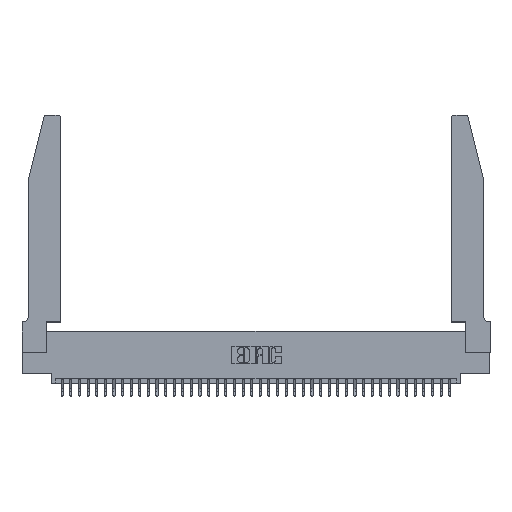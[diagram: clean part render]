
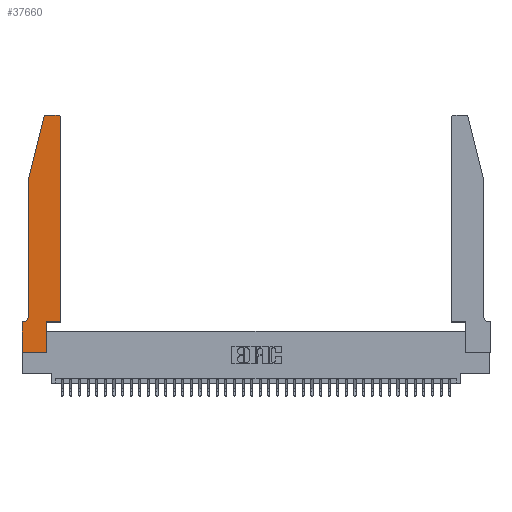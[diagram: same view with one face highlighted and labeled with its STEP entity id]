
A CAD part, top view. The second image highlights one B-rep face of the part: STEP entity #37660.
In plain terms, the highlighted planar face has unit normal (0, 0, 1).
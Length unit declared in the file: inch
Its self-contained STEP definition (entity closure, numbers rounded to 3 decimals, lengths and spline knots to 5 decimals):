
#400 = EDGE_CURVE ( 'NONE', #38491, #24697, #34433, .T. ) ;
#1029 = ORIENTED_EDGE ( 'NONE', *, *, #28770, .T. ) ;
#1080 = LINE ( 'NONE', #39253, #33537 ) ;
#1335 = ORIENTED_EDGE ( 'NONE', *, *, #400, .T. ) ;
#1460 = EDGE_CURVE ( 'NONE', #26523, #8110, #8749, .T. ) ;
#1793 = CIRCLE ( 'NONE', #32976, 0.03 ) ;
#2580 = DIRECTION ( 'NONE',  ( -1., 0., 0. ) ) ;
#3582 = ORIENTED_EDGE ( 'NONE', *, *, #23588, .T. ) ;
#4077 = CARTESIAN_POINT ( 'NONE',  ( 0.284, 2.75, 0.37 ) ) ;
#4135 = LINE ( 'NONE', #27536, #13419 ) ;
#4335 = VERTEX_POINT ( 'NONE', #8247 ) ;
#4940 = CARTESIAN_POINT ( 'NONE',  ( 0., 0., 0.37 ) ) ;
#5087 = ORIENTED_EDGE ( 'NONE', *, *, #16750, .T. ) ;
#5762 = DIRECTION ( 'NONE',  ( 0., 1., 0. ) ) ;
#6700 = CARTESIAN_POINT ( 'NONE',  ( 0.25487, 2.72718, 0.37 ) ) ;
#7778 = EDGE_CURVE ( 'NONE', #38697, #26523, #26146, .T. ) ;
#8110 = VERTEX_POINT ( 'NONE', #27173 ) ;
#8247 = CARTESIAN_POINT ( 'NONE',  ( 0., 0.35, 0.37 ) ) ;
#8749 = LINE ( 'NONE', #33118, #11166 ) ;
#8798 = EDGE_CURVE ( 'NONE', #30592, #4335, #38366, .T. ) ;
#8995 = CARTESIAN_POINT ( 'NONE',  ( 0., 0., 0.37 ) ) ;
#9205 = VERTEX_POINT ( 'NONE', #36816 ) ;
#9849 = ORIENTED_EDGE ( 'NONE', *, *, #14653, .T. ) ;
#10394 = VECTOR ( 'NONE', #10455, 39.37008 ) ;
#10455 = DIRECTION ( 'NONE',  ( 0., -1., 0. ) ) ;
#10794 = DIRECTION ( 'NONE',  ( -1., 0., 0. ) ) ;
#11007 = EDGE_CURVE ( 'NONE', #28979, #38697, #1793, .T. ) ;
#11166 = VECTOR ( 'NONE', #23547, 39.37008 ) ;
#11453 = EDGE_CURVE ( 'NONE', #8110, #30592, #21383, .T. ) ;
#11555 = CARTESIAN_POINT ( 'NONE',  ( 0.2865, 0.35, 0.37 ) ) ;
#11758 = AXIS2_PLACEMENT_3D ( 'NONE', #34910, #22427, #25447 ) ;
#12057 = CARTESIAN_POINT ( 'NONE',  ( 0.2865, 0., 0.37 ) ) ;
#12674 = FACE_OUTER_BOUND ( 'NONE', #14682, .T. ) ;
#12895 = VECTOR ( 'NONE', #31483, 39.37008 ) ;
#13020 = VECTOR ( 'NONE', #16744, 39.37008 ) ;
#13419 = VECTOR ( 'NONE', #37011, 39.37008 ) ;
#14029 = CIRCLE ( 'NONE', #29671, 0.03 ) ;
#14653 = EDGE_CURVE ( 'NONE', #24274, #9205, #23432, .T. ) ;
#14658 = DIRECTION ( 'NONE',  ( 1., 0., 0. ) ) ;
#14682 = EDGE_LOOP ( 'NONE', ( #5087, #16152, #26184, #20063, #27325, #28526, #3582, #1029, #1335, #25719, #9849, #16542 ) ) ;
#14795 = DIRECTION ( 'NONE',  ( -1., 0., 0. ) ) ;
#14952 = CARTESIAN_POINT ( 'NONE',  ( 0.2865, 0.35, 0.37 ) ) ;
#16152 = ORIENTED_EDGE ( 'NONE', *, *, #11007, .T. ) ;
#16542 = ORIENTED_EDGE ( 'NONE', *, *, #33596, .T. ) ;
#16744 = DIRECTION ( 'NONE',  ( 0., 1., 0. ) ) ;
#16750 = EDGE_CURVE ( 'NONE', #25985, #28979, #1080, .T. ) ;
#16856 = CARTESIAN_POINT ( 'NONE',  ( 0.0755, 2., 0.37 ) ) ;
#17897 = CARTESIAN_POINT ( 'NONE',  ( 0.0055, 0.42, 0.37 ) ) ;
#19773 = CARTESIAN_POINT ( 'NONE',  ( 0.0755, 2., 0.37 ) ) ;
#20063 = ORIENTED_EDGE ( 'NONE', *, *, #1460, .T. ) ;
#21276 = CARTESIAN_POINT ( 'NONE',  ( 0.4505, 0.35, 0.37 ) ) ;
#21383 = CIRCLE ( 'NONE', #31456, 0.07 ) ;
#22427 = DIRECTION ( 'NONE',  ( 0., 0., 1. ) ) ;
#22619 = CARTESIAN_POINT ( 'NONE',  ( 0., 0., 0.37 ) ) ;
#22829 = VERTEX_POINT ( 'NONE', #4940 ) ;
#22874 = CARTESIAN_POINT ( 'NONE',  ( 0.284, 2.72, 0.37 ) ) ;
#23319 = DIRECTION ( 'NONE',  ( 0., 0., 1. ) ) ;
#23432 = LINE ( 'NONE', #35628, #13020 ) ;
#23547 = DIRECTION ( 'NONE',  ( 0., -1., 0. ) ) ;
#23588 = EDGE_CURVE ( 'NONE', #4335, #22829, #27208, .T. ) ;
#24274 = VERTEX_POINT ( 'NONE', #21276 ) ;
#24697 = VERTEX_POINT ( 'NONE', #11555 ) ;
#25447 = DIRECTION ( 'NONE',  ( 1., 0., 0. ) ) ;
#25719 = ORIENTED_EDGE ( 'NONE', *, *, #40492, .T. ) ;
#25985 = VERTEX_POINT ( 'NONE', #27115 ) ;
#26146 = LINE ( 'NONE', #16856, #38913 ) ;
#26184 = ORIENTED_EDGE ( 'NONE', *, *, #7778, .T. ) ;
#26523 = VERTEX_POINT ( 'NONE', #19773 ) ;
#27115 = CARTESIAN_POINT ( 'NONE',  ( 0.4205, 2.75, 0.37 ) ) ;
#27173 = CARTESIAN_POINT ( 'NONE',  ( 0.0755, 0.42, 0.37 ) ) ;
#27208 = LINE ( 'NONE', #22619, #10394 ) ;
#27325 = ORIENTED_EDGE ( 'NONE', *, *, #11453, .T. ) ;
#27536 = CARTESIAN_POINT ( 'NONE',  ( 0.4505, 0.35, 0.37 ) ) ;
#28526 = ORIENTED_EDGE ( 'NONE', *, *, #8798, .T. ) ;
#28724 = LINE ( 'NONE', #8995, #12895 ) ;
#28770 = EDGE_CURVE ( 'NONE', #22829, #38491, #28724, .T. ) ;
#28979 = VERTEX_POINT ( 'NONE', #4077 ) ;
#29671 = AXIS2_PLACEMENT_3D ( 'NONE', #33631, #33495, #14658 ) ;
#30006 = VECTOR ( 'NONE', #14795, 39.37008 ) ;
#30063 = DIRECTION ( 'NONE',  ( 0., 0., -1. ) ) ;
#30592 = VERTEX_POINT ( 'NONE', #39988 ) ;
#31456 = AXIS2_PLACEMENT_3D ( 'NONE', #17897, #30063, #10794 ) ;
#31483 = DIRECTION ( 'NONE',  ( 1., 0., 0. ) ) ;
#32480 = DIRECTION ( 'NONE',  ( 1., 0., 0. ) ) ;
#32492 = VECTOR ( 'NONE', #5762, 39.37008 ) ;
#32976 = AXIS2_PLACEMENT_3D ( 'NONE', #22874, #23319, #32480 ) ;
#33118 = CARTESIAN_POINT ( 'NONE',  ( 0.0755, 2., 0.37 ) ) ;
#33495 = DIRECTION ( 'NONE',  ( 0., 0., 1. ) ) ;
#33537 = VECTOR ( 'NONE', #2580, 39.37008 ) ;
#33596 = EDGE_CURVE ( 'NONE', #9205, #25985, #14029, .T. ) ;
#33631 = CARTESIAN_POINT ( 'NONE',  ( 0.4205, 2.72, 0.37 ) ) ;
#33635 = CARTESIAN_POINT ( 'NONE',  ( 0.0755, 0.35, 0.37 ) ) ;
#34433 = LINE ( 'NONE', #14952, #32492 ) ;
#34910 = CARTESIAN_POINT ( 'NONE',  ( 0., 0.35, 0.37 ) ) ;
#35628 = CARTESIAN_POINT ( 'NONE',  ( 0.4505, 0.35, 0.37 ) ) ;
#36816 = CARTESIAN_POINT ( 'NONE',  ( 0.4505, 2.72, 0.37 ) ) ;
#37011 = DIRECTION ( 'NONE',  ( 1., 0., 0. ) ) ;
#37660 = ADVANCED_FACE ( 'NONE', ( #12674 ), #38232, .T. ) ;
#38232 = PLANE ( 'NONE',  #11758 ) ;
#38366 = LINE ( 'NONE', #33635, #30006 ) ;
#38491 = VERTEX_POINT ( 'NONE', #12057 ) ;
#38697 = VERTEX_POINT ( 'NONE', #6700 ) ;
#38913 = VECTOR ( 'NONE', #40640, 39.37008 ) ;
#39253 = CARTESIAN_POINT ( 'NONE',  ( 0.2605, 2.75, 0.37 ) ) ;
#39988 = CARTESIAN_POINT ( 'NONE',  ( 0.0055, 0.35, 0.37 ) ) ;
#40492 = EDGE_CURVE ( 'NONE', #24697, #24274, #4135, .T. ) ;
#40640 = DIRECTION ( 'NONE',  ( -0.239, -0.971, 0. ) ) ;
